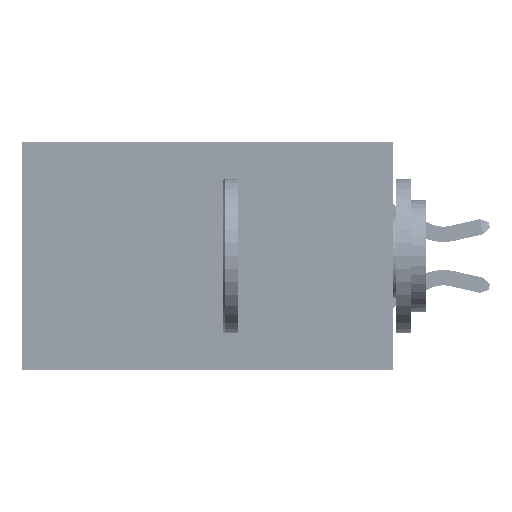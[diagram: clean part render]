
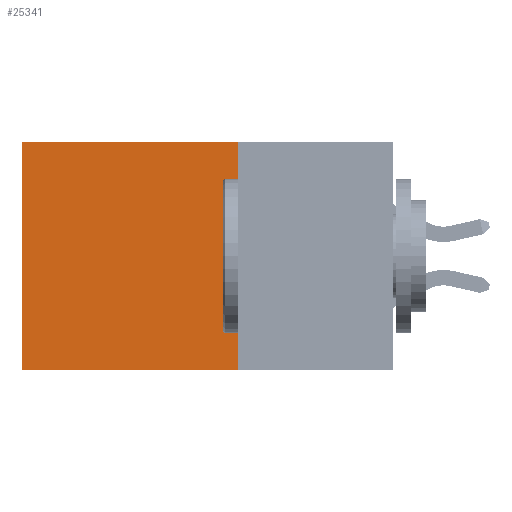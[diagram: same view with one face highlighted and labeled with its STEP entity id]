
A CAD part, left-side view. The second image highlights one B-rep face of the part: STEP entity #25341.
In plain terms, the highlighted planar face has unit normal (-1, 0, 0).
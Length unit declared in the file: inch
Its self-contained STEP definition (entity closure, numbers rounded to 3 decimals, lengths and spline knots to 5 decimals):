
#1490 = CARTESIAN_POINT ( 'NONE',  ( 0.2875, 0.25, -0.37 ) ) ;
#3325 = EDGE_CURVE ( 'NONE', #39484, #30800, #6765, .T. ) ;
#3592 = CARTESIAN_POINT ( 'NONE',  ( 0.2875, 0.6, 0. ) ) ;
#3891 = CARTESIAN_POINT ( 'NONE',  ( 0.2875, 0.25, -0.37 ) ) ;
#4972 = DIRECTION ( 'NONE',  ( 0., 0., -1. ) ) ;
#5521 = EDGE_CURVE ( 'NONE', #36835, #39484, #26724, .T. ) ;
#6765 = LINE ( 'NONE', #3891, #43514 ) ;
#7970 = PLANE ( 'NONE',  #28298 ) ;
#8387 = CARTESIAN_POINT ( 'NONE',  ( 0.2875, 0.6, -0.37 ) ) ;
#8994 = ORIENTED_EDGE ( 'NONE', *, *, #19178, .T. ) ;
#11620 = DIRECTION ( 'NONE',  ( 1., 0., 0. ) ) ;
#16363 = DIRECTION ( 'NONE',  ( 0., 1., 0. ) ) ;
#18672 = CARTESIAN_POINT ( 'NONE',  ( 0.2875, 0.25, 0. ) ) ;
#19178 = EDGE_CURVE ( 'NONE', #45480, #30800, #31871, .T. ) ;
#19938 = EDGE_LOOP ( 'NONE', ( #8994, #20245, #38919, #44398 ) ) ;
#20245 = ORIENTED_EDGE ( 'NONE', *, *, #3325, .F. ) ;
#22820 = CARTESIAN_POINT ( 'NONE',  ( 0.2875, 0.25, 0. ) ) ;
#25341 = ADVANCED_FACE ( 'NONE', ( #32458 ), #7970, .F. ) ;
#26724 = LINE ( 'NONE', #22820, #33944 ) ;
#28298 = AXIS2_PLACEMENT_3D ( 'NONE', #18672, #11620, #36576 ) ;
#28917 = DIRECTION ( 'NONE',  ( 0., 1., 0. ) ) ;
#30800 = VERTEX_POINT ( 'NONE', #8387 ) ;
#31621 = LINE ( 'NONE', #37703, #41046 ) ;
#31871 = LINE ( 'NONE', #45817, #40204 ) ;
#32458 = FACE_OUTER_BOUND ( 'NONE', #19938, .T. ) ;
#33944 = VECTOR ( 'NONE', #4972, 39.37008 ) ;
#35179 = EDGE_CURVE ( 'NONE', #36835, #45480, #31621, .T. ) ;
#35221 = DIRECTION ( 'NONE',  ( 0., 0., -1. ) ) ;
#36576 = DIRECTION ( 'NONE',  ( 0., 0., -1. ) ) ;
#36835 = VERTEX_POINT ( 'NONE', #45831 ) ;
#37703 = CARTESIAN_POINT ( 'NONE',  ( 0.2875, 0.25, 0. ) ) ;
#38919 = ORIENTED_EDGE ( 'NONE', *, *, #5521, .F. ) ;
#39484 = VERTEX_POINT ( 'NONE', #1490 ) ;
#40204 = VECTOR ( 'NONE', #35221, 39.37008 ) ;
#41046 = VECTOR ( 'NONE', #16363, 39.37008 ) ;
#43514 = VECTOR ( 'NONE', #28917, 39.37008 ) ;
#44398 = ORIENTED_EDGE ( 'NONE', *, *, #35179, .T. ) ;
#45480 = VERTEX_POINT ( 'NONE', #3592 ) ;
#45817 = CARTESIAN_POINT ( 'NONE',  ( 0.2875, 0.6, 0. ) ) ;
#45831 = CARTESIAN_POINT ( 'NONE',  ( 0.2875, 0.25, 0. ) ) ;
